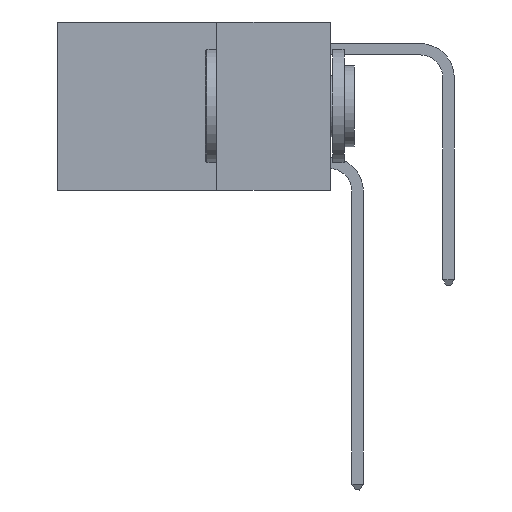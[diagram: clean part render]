
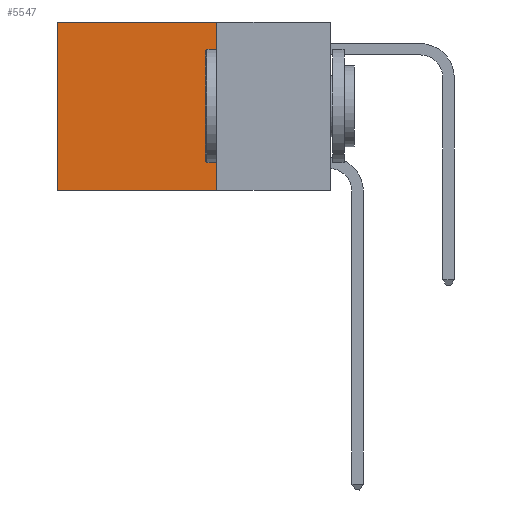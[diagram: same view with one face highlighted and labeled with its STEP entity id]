
A CAD part, left-side view. The second image highlights one B-rep face of the part: STEP entity #5547.
In plain terms, the highlighted planar face has unit normal (-1, 0, 0).
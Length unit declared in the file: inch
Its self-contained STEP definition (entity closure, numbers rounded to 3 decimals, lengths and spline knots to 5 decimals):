
#830 = AXIS2_PLACEMENT_3D ( 'NONE', #1863, #14446, #7650 ) ;
#1236 = VERTEX_POINT ( 'NONE', #9894 ) ;
#1424 = LINE ( 'NONE', #4190, #13267 ) ;
#1538 = CARTESIAN_POINT ( 'NONE',  ( 0.2625, 0.25, -0.37 ) ) ;
#1593 = FACE_OUTER_BOUND ( 'NONE', #12199, .T. ) ;
#1863 = CARTESIAN_POINT ( 'NONE',  ( 0.2625, 0.25, 0. ) ) ;
#2104 = ORIENTED_EDGE ( 'NONE', *, *, #2963, .F. ) ;
#2963 = EDGE_CURVE ( 'NONE', #9359, #10313, #1424, .T. ) ;
#3161 = ORIENTED_EDGE ( 'NONE', *, *, #10947, .F. ) ;
#3910 = ORIENTED_EDGE ( 'NONE', *, *, #9588, .T. ) ;
#4190 = CARTESIAN_POINT ( 'NONE',  ( 0.2625, 0.25, -0.37 ) ) ;
#5346 = DIRECTION ( 'NONE',  ( 0., 1., 0. ) ) ;
#5524 = ORIENTED_EDGE ( 'NONE', *, *, #10242, .T. ) ;
#5547 = ADVANCED_FACE ( 'NONE', ( #1593 ), #11026, .F. ) ;
#6485 = CARTESIAN_POINT ( 'NONE',  ( 0.2625, 0.25, 0. ) ) ;
#6659 = VECTOR ( 'NONE', #11084, 39.37008 ) ;
#7650 = DIRECTION ( 'NONE',  ( 0., 0., -1. ) ) ;
#7681 = DIRECTION ( 'NONE',  ( 0., 1., 0. ) ) ;
#7789 = VERTEX_POINT ( 'NONE', #7898 ) ;
#7898 = CARTESIAN_POINT ( 'NONE',  ( 0.2625, 0.25, 0. ) ) ;
#8757 = VECTOR ( 'NONE', #10010, 39.37008 ) ;
#9240 = VECTOR ( 'NONE', #7681, 39.37008 ) ;
#9359 = VERTEX_POINT ( 'NONE', #1538 ) ;
#9588 = EDGE_CURVE ( 'NONE', #7789, #1236, #12288, .T. ) ;
#9761 = LINE ( 'NONE', #12228, #6659 ) ;
#9894 = CARTESIAN_POINT ( 'NONE',  ( 0.2625, 0.6, 0. ) ) ;
#10010 = DIRECTION ( 'NONE',  ( 0., 0., -1. ) ) ;
#10242 = EDGE_CURVE ( 'NONE', #1236, #10313, #9761, .T. ) ;
#10313 = VERTEX_POINT ( 'NONE', #14547 ) ;
#10947 = EDGE_CURVE ( 'NONE', #7789, #9359, #11798, .T. ) ;
#11026 = PLANE ( 'NONE',  #830 ) ;
#11084 = DIRECTION ( 'NONE',  ( 0., 0., -1. ) ) ;
#11798 = LINE ( 'NONE', #14481, #8757 ) ;
#12199 = EDGE_LOOP ( 'NONE', ( #5524, #2104, #3161, #3910 ) ) ;
#12228 = CARTESIAN_POINT ( 'NONE',  ( 0.2625, 0.6, 0. ) ) ;
#12288 = LINE ( 'NONE', #6485, #9240 ) ;
#13267 = VECTOR ( 'NONE', #5346, 39.37008 ) ;
#14446 = DIRECTION ( 'NONE',  ( 1., 0., 0. ) ) ;
#14481 = CARTESIAN_POINT ( 'NONE',  ( 0.2625, 0.25, 0. ) ) ;
#14547 = CARTESIAN_POINT ( 'NONE',  ( 0.2625, 0.6, -0.37 ) ) ;
